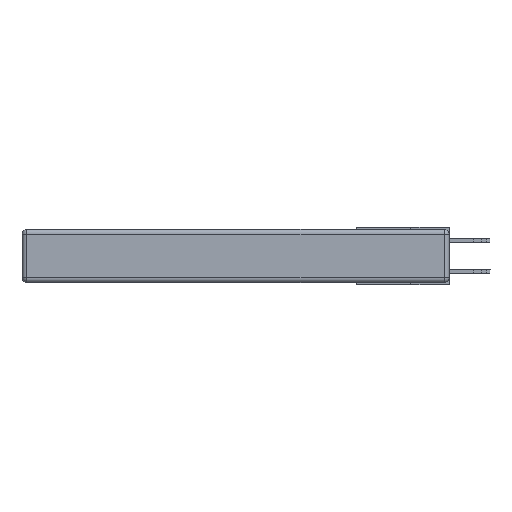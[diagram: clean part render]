
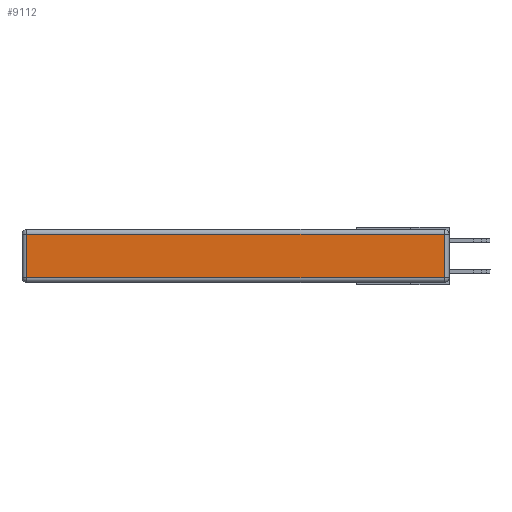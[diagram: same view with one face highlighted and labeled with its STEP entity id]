
A CAD part, left-side view. The second image highlights one B-rep face of the part: STEP entity #9112.
In plain terms, the highlighted planar face has unit normal (-1, 0, 0).
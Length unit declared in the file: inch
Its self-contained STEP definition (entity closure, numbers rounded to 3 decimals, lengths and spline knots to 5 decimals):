
#471 = CARTESIAN_POINT ( 'NONE',  ( 0., 2.72, -0.313 ) ) ;
#625 = EDGE_CURVE ( 'NONE', #9576, #11667, #6339, .T. ) ;
#970 = DIRECTION ( 'NONE',  ( -1., 0., 0. ) ) ;
#1230 = DIRECTION ( 'NONE',  ( 0., 0., -1. ) ) ;
#1395 = CARTESIAN_POINT ( 'NONE',  ( 0., 0., -0.313 ) ) ;
#1461 = EDGE_CURVE ( 'NONE', #10679, #3246, #4414, .T. ) ;
#1671 = VECTOR ( 'NONE', #1230, 39.37008 ) ;
#1937 = CARTESIAN_POINT ( 'NONE',  ( 0., 2.72, -0.343 ) ) ;
#3246 = VERTEX_POINT ( 'NONE', #471 ) ;
#3461 = DIRECTION ( 'NONE',  ( 0., -1., 0. ) ) ;
#3983 = PLANE ( 'NONE',  #4215 ) ;
#3995 = EDGE_CURVE ( 'NONE', #3246, #9576, #6154, .T. ) ;
#4215 = AXIS2_PLACEMENT_3D ( 'NONE', #13183, #970, #12229 ) ;
#4370 = CARTESIAN_POINT ( 'NONE',  ( 0., 2.72, -0.03 ) ) ;
#4414 = LINE ( 'NONE', #1937, #1671 ) ;
#4493 = ORIENTED_EDGE ( 'NONE', *, *, #3995, .T. ) ;
#4909 = FACE_OUTER_BOUND ( 'NONE', #5433, .T. ) ;
#5104 = LINE ( 'NONE', #10018, #7513 ) ;
#5433 = EDGE_LOOP ( 'NONE', ( #4493, #7723, #8847, #7973 ) ) ;
#6154 = LINE ( 'NONE', #1395, #7438 ) ;
#6339 = LINE ( 'NONE', #10742, #7931 ) ;
#7438 = VECTOR ( 'NONE', #3461, 39.37008 ) ;
#7513 = VECTOR ( 'NONE', #10607, 39.37008 ) ;
#7723 = ORIENTED_EDGE ( 'NONE', *, *, #625, .T. ) ;
#7931 = VECTOR ( 'NONE', #12875, 39.37008 ) ;
#7973 = ORIENTED_EDGE ( 'NONE', *, *, #1461, .T. ) ;
#8069 = EDGE_CURVE ( 'NONE', #11667, #10679, #5104, .T. ) ;
#8847 = ORIENTED_EDGE ( 'NONE', *, *, #8069, .T. ) ;
#9112 = ADVANCED_FACE ( 'NONE', ( #4909 ), #3983, .T. ) ;
#9576 = VERTEX_POINT ( 'NONE', #10516 ) ;
#10018 = CARTESIAN_POINT ( 'NONE',  ( 0., 2.75, -0.03 ) ) ;
#10516 = CARTESIAN_POINT ( 'NONE',  ( 0., 0.03, -0.313 ) ) ;
#10607 = DIRECTION ( 'NONE',  ( 0., 1., 0. ) ) ;
#10679 = VERTEX_POINT ( 'NONE', #4370 ) ;
#10742 = CARTESIAN_POINT ( 'NONE',  ( 0., 0.03, -0.343 ) ) ;
#11667 = VERTEX_POINT ( 'NONE', #12754 ) ;
#12229 = DIRECTION ( 'NONE',  ( 0., 0., 1. ) ) ;
#12754 = CARTESIAN_POINT ( 'NONE',  ( 0., 0.03, -0.03 ) ) ;
#12875 = DIRECTION ( 'NONE',  ( 0., 0., 1. ) ) ;
#13183 = CARTESIAN_POINT ( 'NONE',  ( 0., 0., -0.343 ) ) ;
